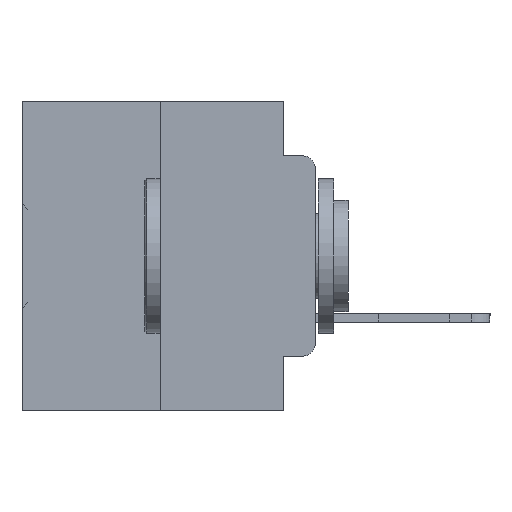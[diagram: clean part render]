
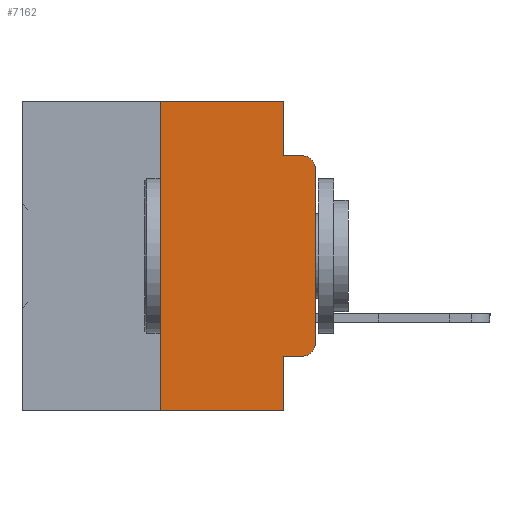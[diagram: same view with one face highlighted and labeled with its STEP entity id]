
A CAD part, left-side view. The second image highlights one B-rep face of the part: STEP entity #7162.
In plain terms, the highlighted planar face has unit normal (-1, 0, 0).
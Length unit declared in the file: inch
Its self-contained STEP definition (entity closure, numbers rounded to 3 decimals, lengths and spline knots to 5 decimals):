
#366 = DIRECTION ( 'NONE',  ( 0., -1., 0. ) ) ;
#897 = CARTESIAN_POINT ( 'NONE',  ( 0., 0.473, -0.5 ) ) ;
#1403 = VECTOR ( 'NONE', #17111, 39.37008 ) ;
#1911 = EDGE_CURVE ( 'NONE', #3115, #32058, #30894, .T. ) ;
#2926 = DIRECTION ( 'NONE',  ( 0., 0., 1. ) ) ;
#3025 = VERTEX_POINT ( 'NONE', #14616 ) ;
#3103 = ORIENTED_EDGE ( 'NONE', *, *, #18482, .F. ) ;
#3115 = VERTEX_POINT ( 'NONE', #3164 ) ;
#3164 = CARTESIAN_POINT ( 'NONE',  ( 0., 0., -0.3915 ) ) ;
#3961 = LINE ( 'NONE', #29069, #25925 ) ;
#4578 = EDGE_CURVE ( 'NONE', #34421, #12186, #3961, .T. ) ;
#4950 = CARTESIAN_POINT ( 'NONE',  ( 0., 0.051, 0. ) ) ;
#6085 = VERTEX_POINT ( 'NONE', #22960 ) ;
#6240 = VERTEX_POINT ( 'NONE', #15591 ) ;
#6427 = VECTOR ( 'NONE', #24197, 39.37008 ) ;
#6448 = LINE ( 'NONE', #34439, #27215 ) ;
#6768 = CARTESIAN_POINT ( 'NONE',  ( 0., 0.25, 0. ) ) ;
#6792 = VECTOR ( 'NONE', #2926, 39.37008 ) ;
#6861 = CARTESIAN_POINT ( 'NONE',  ( 0., 0.051, -0.0885 ) ) ;
#7095 = CARTESIAN_POINT ( 'NONE',  ( 0., 0.25, -0.5 ) ) ;
#7142 = EDGE_CURVE ( 'NONE', #16624, #6240, #36040, .T. ) ;
#7162 = ADVANCED_FACE ( 'NONE', ( #30591 ), #26899, .F. ) ;
#7577 = ORIENTED_EDGE ( 'NONE', *, *, #7608, .T. ) ;
#7608 = EDGE_CURVE ( 'NONE', #9793, #3115, #29740, .T. ) ;
#8406 = LINE ( 'NONE', #6861, #30649 ) ;
#8882 = EDGE_CURVE ( 'NONE', #16624, #34421, #14681, .T. ) ;
#9793 = VERTEX_POINT ( 'NONE', #11339 ) ;
#11339 = CARTESIAN_POINT ( 'NONE',  ( 0., 0.02, -0.4115 ) ) ;
#11379 = CARTESIAN_POINT ( 'NONE',  ( 0., 0., 0. ) ) ;
#11942 = CARTESIAN_POINT ( 'NONE',  ( 0., 0.25, 0. ) ) ;
#12186 = VERTEX_POINT ( 'NONE', #16374 ) ;
#12541 = DIRECTION ( 'NONE',  ( 0., -1., 0. ) ) ;
#12720 = CARTESIAN_POINT ( 'NONE',  ( 0., 0., -0.1085 ) ) ;
#12946 = EDGE_LOOP ( 'NONE', ( #33967, #30152, #17816, #3103, #27819, #23903, #14452, #20872, #22166, #7577 ) ) ;
#13959 = LINE ( 'NONE', #28005, #27726 ) ;
#14452 = ORIENTED_EDGE ( 'NONE', *, *, #7142, .T. ) ;
#14616 = CARTESIAN_POINT ( 'NONE',  ( 0., 0.02, -0.0885 ) ) ;
#14681 = LINE ( 'NONE', #11942, #6792 ) ;
#15591 = CARTESIAN_POINT ( 'NONE',  ( 0., 0.051, -0.5 ) ) ;
#15700 = DIRECTION ( 'NONE',  ( 0., -1., 0. ) ) ;
#15825 = LINE ( 'NONE', #4950, #16675 ) ;
#16035 = DIRECTION ( 'NONE',  ( -1., 0., 0. ) ) ;
#16374 = CARTESIAN_POINT ( 'NONE',  ( 0., 0.051, 0. ) ) ;
#16624 = VERTEX_POINT ( 'NONE', #7095 ) ;
#16675 = VECTOR ( 'NONE', #22311, 39.37008 ) ;
#16888 = CIRCLE ( 'NONE', #30640, 0.02 ) ;
#17111 = DIRECTION ( 'NONE',  ( 0., 0., 1. ) ) ;
#17233 = DIRECTION ( 'NONE',  ( -1., 0., 0. ) ) ;
#17771 = AXIS2_PLACEMENT_3D ( 'NONE', #29612, #35003, #18783 ) ;
#17816 = ORIENTED_EDGE ( 'NONE', *, *, #24023, .F. ) ;
#18358 = VERTEX_POINT ( 'NONE', #24707 ) ;
#18482 = EDGE_CURVE ( 'NONE', #12186, #6085, #15825, .T. ) ;
#18783 = DIRECTION ( 'NONE',  ( 0., 0., -1. ) ) ;
#20872 = ORIENTED_EDGE ( 'NONE', *, *, #28334, .F. ) ;
#22166 = ORIENTED_EDGE ( 'NONE', *, *, #24667, .T. ) ;
#22311 = DIRECTION ( 'NONE',  ( 0., 0., -1. ) ) ;
#22960 = CARTESIAN_POINT ( 'NONE',  ( 0., 0.051, -0.0885 ) ) ;
#23903 = ORIENTED_EDGE ( 'NONE', *, *, #8882, .F. ) ;
#24023 = EDGE_CURVE ( 'NONE', #6085, #3025, #8406, .T. ) ;
#24197 = DIRECTION ( 'NONE',  ( 0., -1., 0. ) ) ;
#24667 = EDGE_CURVE ( 'NONE', #18358, #9793, #6448, .T. ) ;
#24707 = CARTESIAN_POINT ( 'NONE',  ( 0., 0.051, -0.4115 ) ) ;
#25925 = VECTOR ( 'NONE', #12541, 39.37008 ) ;
#26899 = PLANE ( 'NONE',  #17771 ) ;
#27215 = VECTOR ( 'NONE', #366, 39.37008 ) ;
#27726 = VECTOR ( 'NONE', #33383, 39.37008 ) ;
#27819 = ORIENTED_EDGE ( 'NONE', *, *, #4578, .F. ) ;
#28005 = CARTESIAN_POINT ( 'NONE',  ( 0., 0.051, 0. ) ) ;
#28334 = EDGE_CURVE ( 'NONE', #18358, #6240, #13959, .T. ) ;
#29069 = CARTESIAN_POINT ( 'NONE',  ( 0., 0.473, 0. ) ) ;
#29216 = AXIS2_PLACEMENT_3D ( 'NONE', #32351, #16035, #35056 ) ;
#29432 = EDGE_CURVE ( 'NONE', #32058, #3025, #16888, .T. ) ;
#29612 = CARTESIAN_POINT ( 'NONE',  ( 0., 0.473, 0. ) ) ;
#29740 = CIRCLE ( 'NONE', #29216, 0.02 ) ;
#30152 = ORIENTED_EDGE ( 'NONE', *, *, #29432, .T. ) ;
#30591 = FACE_OUTER_BOUND ( 'NONE', #12946, .T. ) ;
#30640 = AXIS2_PLACEMENT_3D ( 'NONE', #33493, #17233, #36230 ) ;
#30649 = VECTOR ( 'NONE', #15700, 39.37008 ) ;
#30894 = LINE ( 'NONE', #11379, #1403 ) ;
#32058 = VERTEX_POINT ( 'NONE', #12720 ) ;
#32351 = CARTESIAN_POINT ( 'NONE',  ( 0., 0.02, -0.3915 ) ) ;
#33383 = DIRECTION ( 'NONE',  ( 0., 0., -1. ) ) ;
#33493 = CARTESIAN_POINT ( 'NONE',  ( 0., 0.02, -0.1085 ) ) ;
#33967 = ORIENTED_EDGE ( 'NONE', *, *, #1911, .T. ) ;
#34421 = VERTEX_POINT ( 'NONE', #6768 ) ;
#34439 = CARTESIAN_POINT ( 'NONE',  ( 0., 0.051, -0.4115 ) ) ;
#35003 = DIRECTION ( 'NONE',  ( 1., 0., 0. ) ) ;
#35056 = DIRECTION ( 'NONE',  ( 0., 0., -1. ) ) ;
#36040 = LINE ( 'NONE', #897, #6427 ) ;
#36230 = DIRECTION ( 'NONE',  ( 0., 0., -1. ) ) ;
